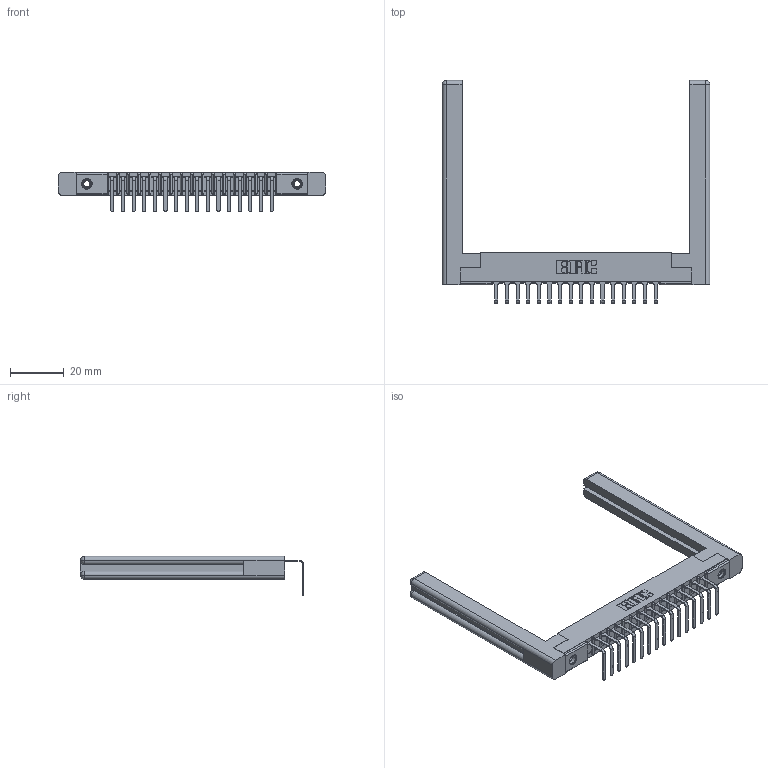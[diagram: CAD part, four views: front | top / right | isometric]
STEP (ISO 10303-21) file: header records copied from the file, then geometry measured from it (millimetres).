
FILE_DESCRIPTION (( 'STEP AP203' ), '1' );
FILE_NAME ('307-016-558-158.STEP', '2019-09-04T12:51:16', ( '' ), ( '' ), 'SwSTEP 2.0', 'SolidWorks 2016', '' );
FILE_SCHEMA (( 'CONFIG_CONTROL_DESIGN' ));
Length unit declared in the file: inch
Products named in the file (5): 307-290-001_558 - 2 (Single); 307-220-058; 345-250-001_345-250-001-102; 307-016-558-158; 307 Part_.156 Dia Mounting Holes
Assembly tree (21 placements, depth 2):
  307-016-558-158
    307 Part_.156 Dia Mounting Holes
    307-290-001_558 - 2 (Single)  x16
    307-220-058  x2
    345-250-001_345-250-001-102  x2
Bounding box: 100.03 x 83.27 x 14.81 mm (x, y, z)
Volume: 14120.3 mm3; surface area: 15475 mm2
Topology: 21 solids, 21 shells, 1237 faces, 3461 edges, 2226 vertices
Faces by surface type: plane 778, cylinder 401, sphere 34, torus 12, cone 12
Entity records: 19659 total; most frequent: CARTESIAN_POINT 3311, ORIENTED_EDGE 3236, DIRECTION 3196, EDGE_CURVE 1618, VECTOR 1226, LINE 1226, VERTEX_POINT 1046, AXIS2_PLACEMENT_3D 985
